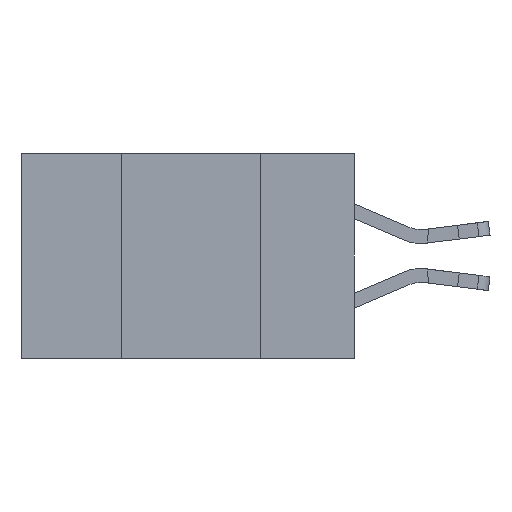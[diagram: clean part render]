
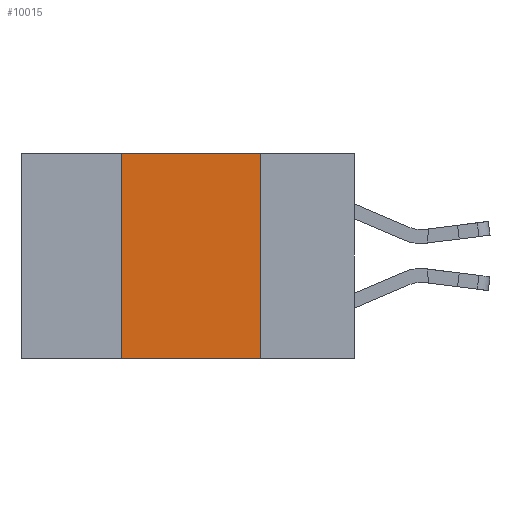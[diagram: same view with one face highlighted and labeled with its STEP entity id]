
A CAD part, left-side view. The second image highlights one B-rep face of the part: STEP entity #10015.
In plain terms, the highlighted planar face has unit normal (-1, 0, 0).
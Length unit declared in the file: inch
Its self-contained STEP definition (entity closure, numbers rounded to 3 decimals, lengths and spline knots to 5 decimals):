
#29 = VECTOR ( 'NONE', #5411, 39.37008 ) ;
#1160 = DIRECTION ( 'NONE',  ( 1., 0., 0. ) ) ;
#1501 = LINE ( 'NONE', #9403, #2107 ) ;
#2107 = VECTOR ( 'NONE', #8411, 39.37008 ) ;
#2526 = CARTESIAN_POINT ( 'NONE',  ( 0., 0.17, -0.37 ) ) ;
#3420 = VERTEX_POINT ( 'NONE', #6157 ) ;
#3504 = ORIENTED_EDGE ( 'NONE', *, *, #10430, .F. ) ;
#3536 = LINE ( 'NONE', #4261, #29 ) ;
#3942 = VERTEX_POINT ( 'NONE', #4359 ) ;
#4090 = VERTEX_POINT ( 'NONE', #2526 ) ;
#4097 = DIRECTION ( 'NONE',  ( 0., 0., -1. ) ) ;
#4114 = CARTESIAN_POINT ( 'NONE',  ( 0., 0.42, -0.37 ) ) ;
#4261 = CARTESIAN_POINT ( 'NONE',  ( 0., 0.42, -0.37 ) ) ;
#4359 = CARTESIAN_POINT ( 'NONE',  ( 0., 0.17, 0. ) ) ;
#5210 = CARTESIAN_POINT ( 'NONE',  ( 0., 0.17, -0.37 ) ) ;
#5411 = DIRECTION ( 'NONE',  ( 0., 0., 1. ) ) ;
#6002 = LINE ( 'NONE', #12646, #8681 ) ;
#6088 = PLANE ( 'NONE',  #7476 ) ;
#6157 = CARTESIAN_POINT ( 'NONE',  ( 0., 0.42, 0. ) ) ;
#6982 = CARTESIAN_POINT ( 'NONE',  ( 0., 0.6, 0. ) ) ;
#7427 = ORIENTED_EDGE ( 'NONE', *, *, #11308, .T. ) ;
#7476 = AXIS2_PLACEMENT_3D ( 'NONE', #6982, #1160, #4097 ) ;
#7705 = EDGE_LOOP ( 'NONE', ( #9491, #3504, #9134, #7427 ) ) ;
#8268 = VECTOR ( 'NONE', #12221, 39.37008 ) ;
#8411 = DIRECTION ( 'NONE',  ( 0., -1., 0. ) ) ;
#8681 = VECTOR ( 'NONE', #11673, 39.37008 ) ;
#9134 = ORIENTED_EDGE ( 'NONE', *, *, #9288, .F. ) ;
#9288 = EDGE_CURVE ( 'NONE', #11170, #3420, #3536, .T. ) ;
#9403 = CARTESIAN_POINT ( 'NONE',  ( 0., 0.6, -0.37 ) ) ;
#9491 = ORIENTED_EDGE ( 'NONE', *, *, #9686, .F. ) ;
#9686 = EDGE_CURVE ( 'NONE', #3942, #4090, #10165, .T. ) ;
#10015 = ADVANCED_FACE ( 'NONE', ( #11943 ), #6088, .F. ) ;
#10165 = LINE ( 'NONE', #5210, #8268 ) ;
#10430 = EDGE_CURVE ( 'NONE', #3420, #3942, #6002, .T. ) ;
#11170 = VERTEX_POINT ( 'NONE', #4114 ) ;
#11308 = EDGE_CURVE ( 'NONE', #11170, #4090, #1501, .T. ) ;
#11673 = DIRECTION ( 'NONE',  ( 0., -1., 0. ) ) ;
#11943 = FACE_OUTER_BOUND ( 'NONE', #7705, .T. ) ;
#12221 = DIRECTION ( 'NONE',  ( 0., 0., -1. ) ) ;
#12646 = CARTESIAN_POINT ( 'NONE',  ( 0., 0.6, 0. ) ) ;
